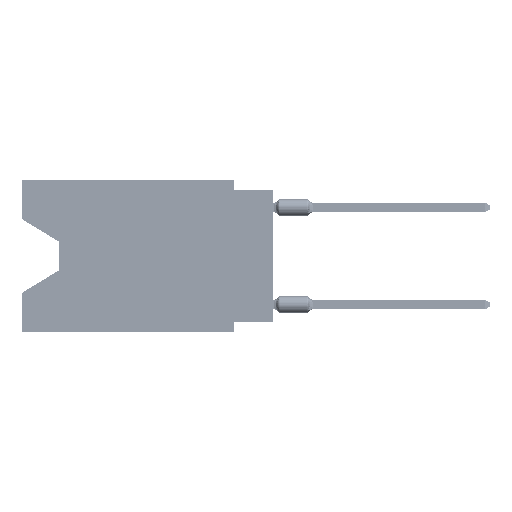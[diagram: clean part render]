
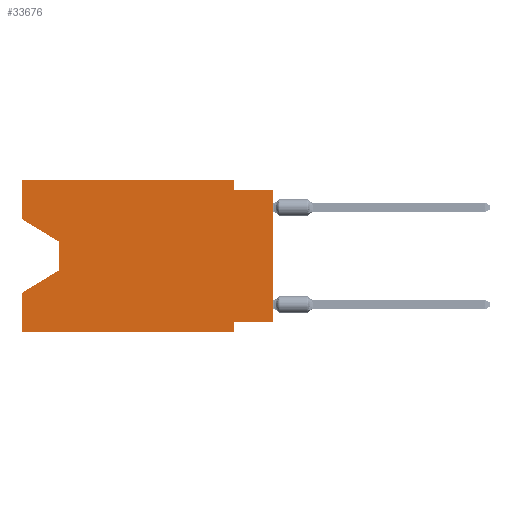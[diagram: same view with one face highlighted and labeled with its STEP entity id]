
A CAD part, left-side view. The second image highlights one B-rep face of the part: STEP entity #33676.
In plain terms, the highlighted planar face has unit normal (-1, 0, 0).
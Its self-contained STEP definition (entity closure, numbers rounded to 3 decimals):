
#412 = ORIENTED_EDGE ( 'NONE', *, *, #11980, .T. ) ;
#1543 = CARTESIAN_POINT ( 'NONE',  ( 0., 2.54, -9.906 ) ) ;
#1704 = ORIENTED_EDGE ( 'NONE', *, *, #10378, .F. ) ;
#2592 = ORIENTED_EDGE ( 'NONE', *, *, #54842, .F. ) ;
#3710 = CARTESIAN_POINT ( 'NONE',  ( 0., 0., -9.271 ) ) ;
#4226 = CARTESIAN_POINT ( 'NONE',  ( 0., 0., 0. ) ) ;
#6150 = CARTESIAN_POINT ( 'NONE',  ( 0., 13.97, -4.013 ) ) ;
#8127 = VECTOR ( 'NONE', #74653, 1000. ) ;
#8258 = PLANE ( 'NONE',  #49826 ) ;
#9145 = EDGE_CURVE ( 'NONE', #39235, #69033, #43284, .T. ) ;
#9889 = CARTESIAN_POINT ( 'NONE',  ( 0., 16.383, 0. ) ) ;
#10048 = DIRECTION ( 'NONE',  ( 0., -1., 0. ) ) ;
#10083 = DIRECTION ( 'NONE',  ( 0., 0., 1. ) ) ;
#10378 = EDGE_CURVE ( 'NONE', #48335, #52314, #67513, .T. ) ;
#11848 = VECTOR ( 'NONE', #13294, 1000. ) ;
#11980 = EDGE_CURVE ( 'NONE', #60138, #74286, #32052, .T. ) ;
#13294 = DIRECTION ( 'NONE',  ( 0., -0.855, -0.519 ) ) ;
#14805 = DIRECTION ( 'NONE',  ( 0., -1., 0. ) ) ;
#15535 = DIRECTION ( 'NONE',  ( 0., 0., -1. ) ) ;
#15664 = DIRECTION ( 'NONE',  ( 0., 0., 1. ) ) ;
#18000 = VECTOR ( 'NONE', #14805, 1000. ) ;
#18467 = EDGE_CURVE ( 'NONE', #55211, #22818, #32972, .T. ) ;
#19792 = DIRECTION ( 'NONE',  ( 1., 0., 0. ) ) ;
#21568 = VERTEX_POINT ( 'NONE', #27460 ) ;
#21859 = CARTESIAN_POINT ( 'NONE',  ( 0., 13.97, -5.893 ) ) ;
#22559 = ORIENTED_EDGE ( 'NONE', *, *, #68044, .F. ) ;
#22818 = VERTEX_POINT ( 'NONE', #49175 ) ;
#24005 = VECTOR ( 'NONE', #10083, 1000. ) ;
#25838 = ORIENTED_EDGE ( 'NONE', *, *, #31886, .F. ) ;
#25872 = CARTESIAN_POINT ( 'NONE',  ( 0., 16.383, -7.36 ) ) ;
#26663 = VERTEX_POINT ( 'NONE', #25872 ) ;
#27194 = DIRECTION ( 'NONE',  ( 0., 1., 0. ) ) ;
#27460 = CARTESIAN_POINT ( 'NONE',  ( 0., 16.383, 0. ) ) ;
#27641 = CARTESIAN_POINT ( 'NONE',  ( 0., 0., -9.271 ) ) ;
#28344 = LINE ( 'NONE', #70273, #76013 ) ;
#29015 = ORIENTED_EDGE ( 'NONE', *, *, #61732, .T. ) ;
#29653 = DIRECTION ( 'NONE',  ( 0., 0., -1. ) ) ;
#30012 = VECTOR ( 'NONE', #15664, 1000. ) ;
#30994 = ORIENTED_EDGE ( 'NONE', *, *, #63512, .T. ) ;
#31159 = ORIENTED_EDGE ( 'NONE', *, *, #61497, .T. ) ;
#31567 = CARTESIAN_POINT ( 'NONE',  ( 0., 2.54, 0. ) ) ;
#31735 = FACE_OUTER_BOUND ( 'NONE', #60190, .T. ) ;
#31886 = EDGE_CURVE ( 'NONE', #39235, #21568, #38009, .T. ) ;
#32052 = LINE ( 'NONE', #55910, #59933 ) ;
#32120 = CARTESIAN_POINT ( 'NONE',  ( 0., 0., -0.635 ) ) ;
#32475 = CARTESIAN_POINT ( 'NONE',  ( 0., 16.383, 0. ) ) ;
#32972 = LINE ( 'NONE', #3710, #54814 ) ;
#33676 = ADVANCED_FACE ( 'NONE', ( #31735 ), #8258, .F. ) ;
#33733 = DIRECTION ( 'NONE',  ( 0., 0.855, -0.519 ) ) ;
#37069 = DIRECTION ( 'NONE',  ( 0., -1., 0. ) ) ;
#37207 = ORIENTED_EDGE ( 'NONE', *, *, #18467, .F. ) ;
#37793 = EDGE_CURVE ( 'NONE', #22818, #74286, #46982, .T. ) ;
#38009 = LINE ( 'NONE', #9889, #30012 ) ;
#39180 = VERTEX_POINT ( 'NONE', #31567 ) ;
#39235 = VERTEX_POINT ( 'NONE', #73102 ) ;
#40046 = CARTESIAN_POINT ( 'NONE',  ( 0., 2.54, -9.906 ) ) ;
#41275 = ORIENTED_EDGE ( 'NONE', *, *, #37793, .F. ) ;
#43284 = LINE ( 'NONE', #49071, #11848 ) ;
#44180 = VECTOR ( 'NONE', #10048, 1000. ) ;
#45214 = VERTEX_POINT ( 'NONE', #21859 ) ;
#45447 = LINE ( 'NONE', #63532, #44180 ) ;
#46982 = LINE ( 'NONE', #1543, #54993 ) ;
#48335 = VERTEX_POINT ( 'NONE', #70764 ) ;
#49071 = CARTESIAN_POINT ( 'NONE',  ( 0., 16.383, -2.546 ) ) ;
#49175 = CARTESIAN_POINT ( 'NONE',  ( 0., 2.54, -9.271 ) ) ;
#49282 = VECTOR ( 'NONE', #51243, 1000. ) ;
#49826 = AXIS2_PLACEMENT_3D ( 'NONE', #32475, #19792, #15535 ) ;
#51243 = DIRECTION ( 'NONE',  ( 0., 0., -1. ) ) ;
#52314 = VERTEX_POINT ( 'NONE', #69990 ) ;
#52396 = CARTESIAN_POINT ( 'NONE',  ( 0., 2.54, 0. ) ) ;
#53102 = LINE ( 'NONE', #6150, #67108 ) ;
#54798 = CARTESIAN_POINT ( 'NONE',  ( 0., 13.97, -4.013 ) ) ;
#54814 = VECTOR ( 'NONE', #27194, 1000. ) ;
#54842 = EDGE_CURVE ( 'NONE', #21568, #39180, #45447, .T. ) ;
#54993 = VECTOR ( 'NONE', #29653, 1000. ) ;
#55157 = LINE ( 'NONE', #56654, #24005 ) ;
#55211 = VERTEX_POINT ( 'NONE', #27641 ) ;
#55910 = CARTESIAN_POINT ( 'NONE',  ( 0., 16.383, -9.906 ) ) ;
#56654 = CARTESIAN_POINT ( 'NONE',  ( 0., 16.383, 0. ) ) ;
#57363 = DIRECTION ( 'NONE',  ( 0., 0., -1. ) ) ;
#58685 = EDGE_CURVE ( 'NONE', #60138, #26663, #55157, .T. ) ;
#59933 = VECTOR ( 'NONE', #37069, 1000. ) ;
#60122 = LINE ( 'NONE', #4226, #8127 ) ;
#60138 = VERTEX_POINT ( 'NONE', #68945 ) ;
#60190 = EDGE_LOOP ( 'NONE', ( #67892, #29015, #30994, #72026, #412, #41275, #37207, #31159, #1704, #22559, #2592, #25838 ) ) ;
#61497 = EDGE_CURVE ( 'NONE', #55211, #52314, #60122, .T. ) ;
#61732 = EDGE_CURVE ( 'NONE', #69033, #45214, #53102, .T. ) ;
#63512 = EDGE_CURVE ( 'NONE', #45214, #26663, #28344, .T. ) ;
#63532 = CARTESIAN_POINT ( 'NONE',  ( 0., 16.383, 0. ) ) ;
#67108 = VECTOR ( 'NONE', #57363, 1000. ) ;
#67513 = LINE ( 'NONE', #32120, #18000 ) ;
#67892 = ORIENTED_EDGE ( 'NONE', *, *, #9145, .T. ) ;
#68044 = EDGE_CURVE ( 'NONE', #39180, #48335, #74709, .T. ) ;
#68945 = CARTESIAN_POINT ( 'NONE',  ( 0., 16.383, -9.906 ) ) ;
#69033 = VERTEX_POINT ( 'NONE', #54798 ) ;
#69990 = CARTESIAN_POINT ( 'NONE',  ( 0., 0., -0.635 ) ) ;
#70273 = CARTESIAN_POINT ( 'NONE',  ( 0., 13.97, -5.893 ) ) ;
#70764 = CARTESIAN_POINT ( 'NONE',  ( 0., 2.54, -0.635 ) ) ;
#72026 = ORIENTED_EDGE ( 'NONE', *, *, #58685, .F. ) ;
#73102 = CARTESIAN_POINT ( 'NONE',  ( 0., 16.383, -2.546 ) ) ;
#74286 = VERTEX_POINT ( 'NONE', #40046 ) ;
#74653 = DIRECTION ( 'NONE',  ( 0., 0., 1. ) ) ;
#74709 = LINE ( 'NONE', #52396, #49282 ) ;
#76013 = VECTOR ( 'NONE', #33733, 1000. ) ;
